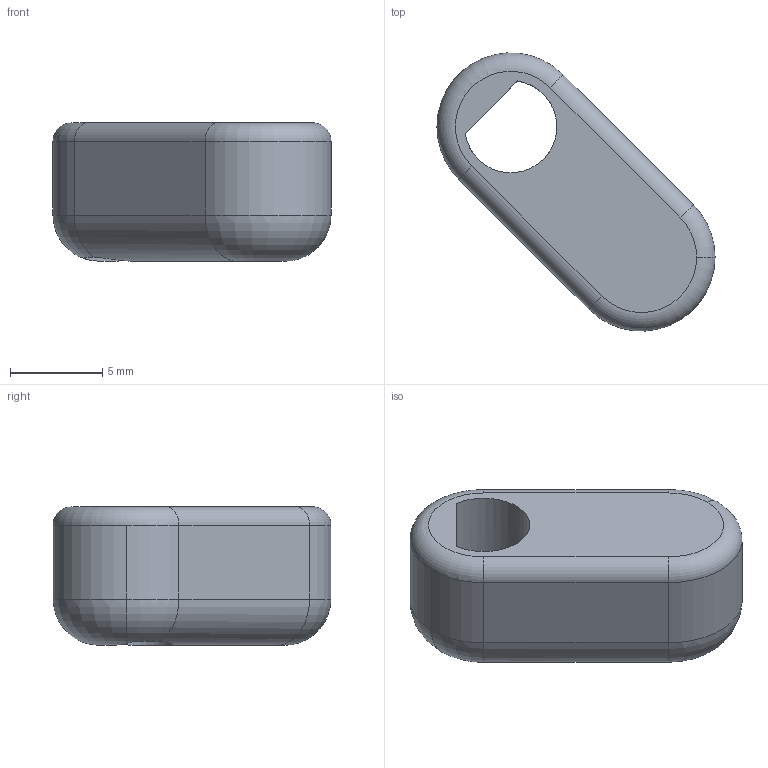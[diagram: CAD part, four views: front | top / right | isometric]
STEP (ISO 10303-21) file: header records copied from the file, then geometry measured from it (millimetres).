
FILE_DESCRIPTION (( 'STEP AP214' ), '1' );
FILE_NAME ('Mag_Release_Right.step', '2014-05-14T06:09:39', ( 'WarFairy' ), ( '' ), 'SwSTEP 2.0', 'SolidWorks 2013', '' );
FILE_SCHEMA (( 'AUTOMOTIVE_DESIGN' ));
Length unit declared in the file: inch
Products named in the file (1): Mag_Release_Right
Bounding box: 15.07 x 15.06 x 7.5 mm (x, y, z)
Volume: 785.8 mm3; surface area: 605.8 mm2
Topology: 1 solids, 1 shells, 21 faces, 49 edges, 29 vertices
Faces by surface type: cylinder 9, torus 7, plane 5
Entity records: 667 total; most frequent: CARTESIAN_POINT 128, DIRECTION 117, ORIENTED_EDGE 98, AXIS2_PLACEMENT_3D 50, EDGE_CURVE 49, VERTEX_POINT 29, CIRCLE 28, EDGE_LOOP 22
